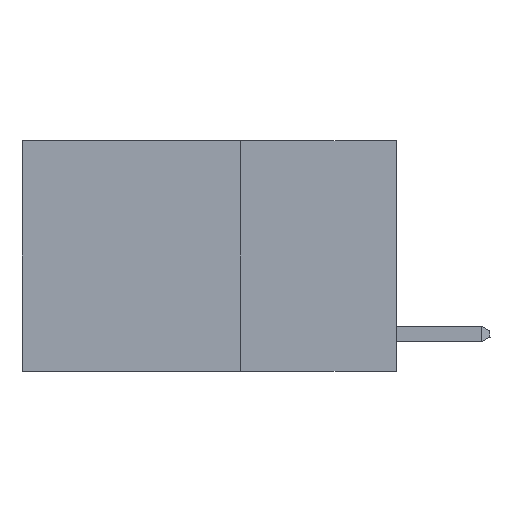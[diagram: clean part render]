
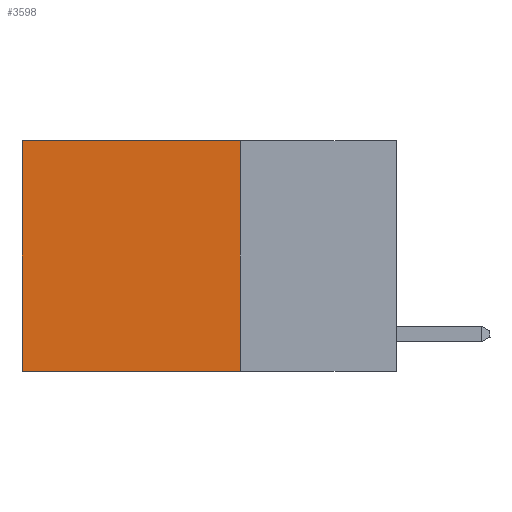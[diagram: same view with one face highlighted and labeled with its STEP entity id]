
A CAD part, left-side view. The second image highlights one B-rep face of the part: STEP entity #3598.
In plain terms, the highlighted planar face has unit normal (-1, 0, 0).
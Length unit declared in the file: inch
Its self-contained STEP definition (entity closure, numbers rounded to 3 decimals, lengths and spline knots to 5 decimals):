
#75 = CARTESIAN_POINT ( 'NONE',  ( 0.2625, 0.6, 0. ) ) ;
#423 = VECTOR ( 'NONE', #5893, 39.37008 ) ;
#707 = CARTESIAN_POINT ( 'NONE',  ( 0.2625, 0.25, 0. ) ) ;
#1039 = LINE ( 'NONE', #3563, #8971 ) ;
#1636 = ORIENTED_EDGE ( 'NONE', *, *, #4806, .F. ) ;
#2001 = CARTESIAN_POINT ( 'NONE',  ( 0.2625, 0.25, 0. ) ) ;
#2123 = CARTESIAN_POINT ( 'NONE',  ( 0.2625, 0.6, -0.37 ) ) ;
#2124 = ORIENTED_EDGE ( 'NONE', *, *, #7931, .T. ) ;
#2337 = ORIENTED_EDGE ( 'NONE', *, *, #8783, .T. ) ;
#3033 = VECTOR ( 'NONE', #3424, 39.37008 ) ;
#3259 = FACE_OUTER_BOUND ( 'NONE', #7708, .T. ) ;
#3424 = DIRECTION ( 'NONE',  ( 0., 0., -1. ) ) ;
#3563 = CARTESIAN_POINT ( 'NONE',  ( 0.2625, 0.25, 0. ) ) ;
#3598 = ADVANCED_FACE ( 'NONE', ( #3259 ), #10670, .F. ) ;
#4084 = CARTESIAN_POINT ( 'NONE',  ( 0.2625, 0.25, 0. ) ) ;
#4089 = DIRECTION ( 'NONE',  ( 1., 0., 0. ) ) ;
#4655 = DIRECTION ( 'NONE',  ( 0., 1., 0. ) ) ;
#4714 = CARTESIAN_POINT ( 'NONE',  ( 0.2625, 0.25, -0.37 ) ) ;
#4806 = EDGE_CURVE ( 'NONE', #7043, #10574, #9961, .T. ) ;
#5784 = LINE ( 'NONE', #4084, #423 ) ;
#5814 = VERTEX_POINT ( 'NONE', #9581 ) ;
#5826 = VERTEX_POINT ( 'NONE', #2001 ) ;
#5893 = DIRECTION ( 'NONE',  ( 0., 0., -1. ) ) ;
#6661 = DIRECTION ( 'NONE',  ( 0., 0., -1. ) ) ;
#6793 = ORIENTED_EDGE ( 'NONE', *, *, #10695, .F. ) ;
#7043 = VERTEX_POINT ( 'NONE', #10256 ) ;
#7704 = LINE ( 'NONE', #75, #3033 ) ;
#7708 = EDGE_LOOP ( 'NONE', ( #2124, #1636, #6793, #2337 ) ) ;
#7841 = DIRECTION ( 'NONE',  ( 0., 1., 0. ) ) ;
#7931 = EDGE_CURVE ( 'NONE', #5814, #10574, #7704, .T. ) ;
#8783 = EDGE_CURVE ( 'NONE', #5826, #5814, #1039, .T. ) ;
#8971 = VECTOR ( 'NONE', #7841, 39.37008 ) ;
#9581 = CARTESIAN_POINT ( 'NONE',  ( 0.2625, 0.6, 0. ) ) ;
#9961 = LINE ( 'NONE', #4714, #10862 ) ;
#10256 = CARTESIAN_POINT ( 'NONE',  ( 0.2625, 0.25, -0.37 ) ) ;
#10574 = VERTEX_POINT ( 'NONE', #2123 ) ;
#10657 = AXIS2_PLACEMENT_3D ( 'NONE', #707, #4089, #6661 ) ;
#10670 = PLANE ( 'NONE',  #10657 ) ;
#10695 = EDGE_CURVE ( 'NONE', #5826, #7043, #5784, .T. ) ;
#10862 = VECTOR ( 'NONE', #4655, 39.37008 ) ;
